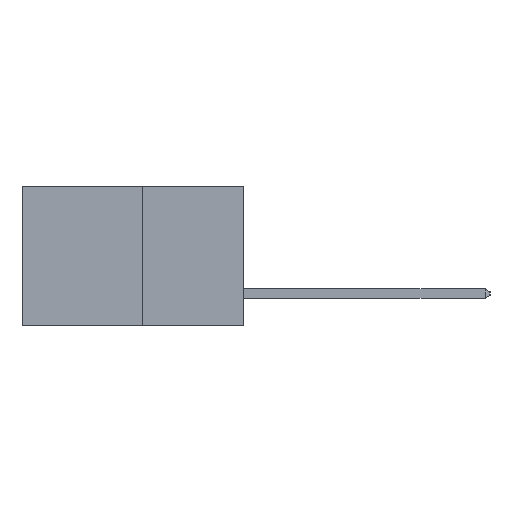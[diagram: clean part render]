
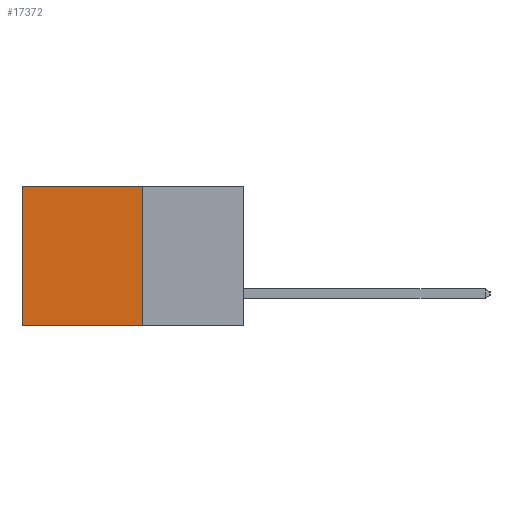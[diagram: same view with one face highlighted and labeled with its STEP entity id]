
A CAD part, left-side view. The second image highlights one B-rep face of the part: STEP entity #17372.
In plain terms, the highlighted planar face has unit normal (-1, 0, 0).
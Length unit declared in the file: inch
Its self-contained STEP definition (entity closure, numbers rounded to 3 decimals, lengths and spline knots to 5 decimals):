
#138 = DIRECTION ( 'NONE',  ( 0., 1., 0. ) ) ;
#222 = CARTESIAN_POINT ( 'NONE',  ( 0.277, 0.59, -0.37 ) ) ;
#664 = ORIENTED_EDGE ( 'NONE', *, *, #5354, .F. ) ;
#741 = CARTESIAN_POINT ( 'NONE',  ( 0.277, 0.59, 0. ) ) ;
#972 = DIRECTION ( 'NONE',  ( 0., 1., 0. ) ) ;
#2049 = EDGE_CURVE ( 'NONE', #11162, #5726, #7322, .T. ) ;
#2551 = CARTESIAN_POINT ( 'NONE',  ( 0.277, 0.27, -0.37 ) ) ;
#3032 = ORIENTED_EDGE ( 'NONE', *, *, #4284, .T. ) ;
#3325 = CARTESIAN_POINT ( 'NONE',  ( 0.277, 0.59, -0.37 ) ) ;
#4284 = EDGE_CURVE ( 'NONE', #12304, #4602, #17495, .T. ) ;
#4602 = VERTEX_POINT ( 'NONE', #741 ) ;
#5233 = CARTESIAN_POINT ( 'NONE',  ( 0.277, 0.27, -0.37 ) ) ;
#5354 = EDGE_CURVE ( 'NONE', #12304, #11162, #11537, .T. ) ;
#5726 = VERTEX_POINT ( 'NONE', #222 ) ;
#6788 = DIRECTION ( 'NONE',  ( 0., 0., -1. ) ) ;
#7322 = LINE ( 'NONE', #18688, #14684 ) ;
#8372 = CARTESIAN_POINT ( 'NONE',  ( 0.277, 0.27, -0.37 ) ) ;
#9687 = LINE ( 'NONE', #3325, #13149 ) ;
#10901 = CARTESIAN_POINT ( 'NONE',  ( 0.277, 0.27, 0. ) ) ;
#11094 = VECTOR ( 'NONE', #17259, 39.37008 ) ;
#11162 = VERTEX_POINT ( 'NONE', #8372 ) ;
#11537 = LINE ( 'NONE', #2551, #11094 ) ;
#12304 = VERTEX_POINT ( 'NONE', #10901 ) ;
#12640 = PLANE ( 'NONE',  #19296 ) ;
#12677 = FACE_OUTER_BOUND ( 'NONE', #18326, .T. ) ;
#13149 = VECTOR ( 'NONE', #15296, 39.37008 ) ;
#13637 = VECTOR ( 'NONE', #972, 39.37008 ) ;
#14684 = VECTOR ( 'NONE', #138, 39.37008 ) ;
#14838 = EDGE_CURVE ( 'NONE', #4602, #5726, #9687, .T. ) ;
#15083 = ORIENTED_EDGE ( 'NONE', *, *, #2049, .F. ) ;
#15132 = ORIENTED_EDGE ( 'NONE', *, *, #14838, .T. ) ;
#15296 = DIRECTION ( 'NONE',  ( 0., 0., -1. ) ) ;
#15623 = DIRECTION ( 'NONE',  ( 1., 0., 0. ) ) ;
#16508 = CARTESIAN_POINT ( 'NONE',  ( 0.277, 0.27, 0. ) ) ;
#17259 = DIRECTION ( 'NONE',  ( 0., 0., -1. ) ) ;
#17372 = ADVANCED_FACE ( 'NONE', ( #12677 ), #12640, .F. ) ;
#17495 = LINE ( 'NONE', #16508, #13637 ) ;
#18326 = EDGE_LOOP ( 'NONE', ( #15132, #15083, #664, #3032 ) ) ;
#18688 = CARTESIAN_POINT ( 'NONE',  ( 0.277, 0.27, -0.37 ) ) ;
#19296 = AXIS2_PLACEMENT_3D ( 'NONE', #5233, #15623, #6788 ) ;
